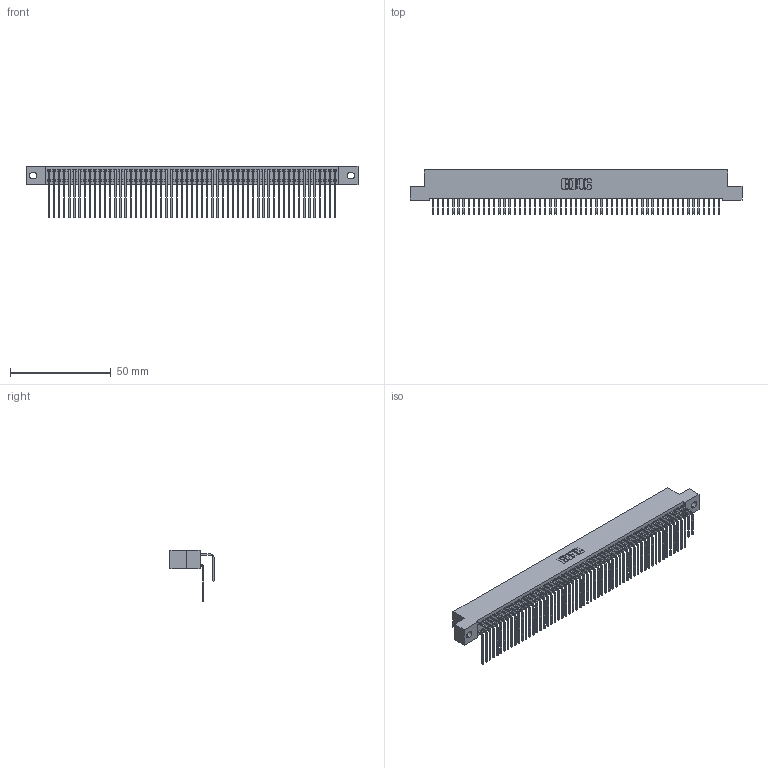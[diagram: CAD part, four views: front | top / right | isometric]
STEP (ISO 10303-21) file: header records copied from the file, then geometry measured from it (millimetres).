
FILE_DESCRIPTION (( 'STEP AP203' ), '1' );
FILE_NAME ('342-114-558-202.STEP', '2019-10-04T21:48:28', ( '' ), ( '' ), 'SwSTEP 2.0', 'SolidWorks 2016', '' );
FILE_SCHEMA (( 'CONFIG_CONTROL_DESIGN' ));
Length unit declared in the file: inch
Products named in the file (4): 342 Part_.128 Slot; 345-292-001_558 559 Tail - 1; 345-292-001_558 Tail - 2; 342-114-558-202
Assembly tree (115 placements, depth 2):
  342-114-558-202
    342 Part_.128 Slot
    345-292-001_558 559 Tail - 1  x57
    345-292-001_558 Tail - 2  x57
Bounding box: 165.1 x 21.91 x 25.78 mm (x, y, z)
Volume: 15510.7 mm3; surface area: 28351.5 mm2
Topology: 115 solids, 115 shells, 6270 faces, 18665 edges, 12290 vertices
Faces by surface type: plane 4402, cylinder 1868
Entity records: 36517 total; most frequent: CARTESIAN_POINT 6085, ORIENTED_EDGE 5970, DIRECTION 5153, EDGE_CURVE 2985, VECTOR 2817, LINE 2817, VERTEX_POINT 1986, AXIS2_PLACEMENT_3D 1168
